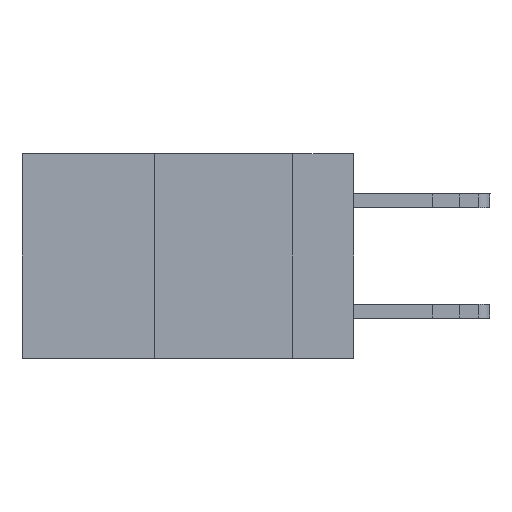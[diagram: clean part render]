
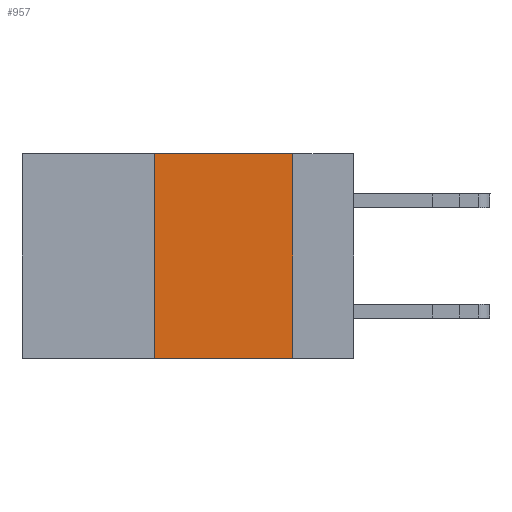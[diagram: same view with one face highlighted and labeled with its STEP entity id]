
A CAD part, left-side view. The second image highlights one B-rep face of the part: STEP entity #957.
In plain terms, the highlighted planar face has unit normal (-1, 0, 0).
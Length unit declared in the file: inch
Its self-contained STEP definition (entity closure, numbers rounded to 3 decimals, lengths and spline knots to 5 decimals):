
#957 = ADVANCED_FACE ( 'NONE', ( #14473 ), #7053, .F. ) ;
#1133 = CARTESIAN_POINT ( 'NONE',  ( 0., 0.36, 0. ) ) ;
#2918 = VERTEX_POINT ( 'NONE', #21353 ) ;
#3142 = EDGE_CURVE ( 'NONE', #7603, #15066, #15410, .T. ) ;
#4010 = EDGE_LOOP ( 'NONE', ( #4540, #5049, #11588, #8796 ) ) ;
#4540 = ORIENTED_EDGE ( 'NONE', *, *, #12472, .F. ) ;
#4547 = LINE ( 'NONE', #1133, #7385 ) ;
#4725 = DIRECTION ( 'NONE',  ( 0., 0., -1. ) ) ;
#4983 = CARTESIAN_POINT ( 'NONE',  ( 0., 0.36, 0. ) ) ;
#5049 = ORIENTED_EDGE ( 'NONE', *, *, #16550, .F. ) ;
#5548 = DIRECTION ( 'NONE',  ( 0., 0., 1. ) ) ;
#5970 = CARTESIAN_POINT ( 'NONE',  ( 0., 0.11, -0.37 ) ) ;
#6630 = VECTOR ( 'NONE', #7827, 39.37008 ) ;
#7053 = PLANE ( 'NONE',  #13541 ) ;
#7385 = VECTOR ( 'NONE', #5548, 39.37008 ) ;
#7603 = VERTEX_POINT ( 'NONE', #17558 ) ;
#7827 = DIRECTION ( 'NONE',  ( 0., -1., 0. ) ) ;
#8043 = VECTOR ( 'NONE', #4725, 39.37008 ) ;
#8620 = CARTESIAN_POINT ( 'NONE',  ( 0., 0.6, 0. ) ) ;
#8796 = ORIENTED_EDGE ( 'NONE', *, *, #3142, .T. ) ;
#9629 = CARTESIAN_POINT ( 'NONE',  ( 0., 0.6, 0. ) ) ;
#11544 = DIRECTION ( 'NONE',  ( 0., -1., 0. ) ) ;
#11588 = ORIENTED_EDGE ( 'NONE', *, *, #17045, .F. ) ;
#12472 = EDGE_CURVE ( 'NONE', #2918, #15066, #12533, .T. ) ;
#12533 = LINE ( 'NONE', #14823, #8043 ) ;
#13541 = AXIS2_PLACEMENT_3D ( 'NONE', #8620, #13663, #15583 ) ;
#13663 = DIRECTION ( 'NONE',  ( 1., 0., 0. ) ) ;
#14473 = FACE_OUTER_BOUND ( 'NONE', #4010, .T. ) ;
#14823 = CARTESIAN_POINT ( 'NONE',  ( 0., 0.11, 0. ) ) ;
#14886 = VECTOR ( 'NONE', #11544, 39.37008 ) ;
#15066 = VERTEX_POINT ( 'NONE', #5970 ) ;
#15377 = LINE ( 'NONE', #9629, #6630 ) ;
#15410 = LINE ( 'NONE', #19911, #14886 ) ;
#15583 = DIRECTION ( 'NONE',  ( 0., 0., -1. ) ) ;
#16550 = EDGE_CURVE ( 'NONE', #17274, #2918, #15377, .T. ) ;
#17045 = EDGE_CURVE ( 'NONE', #7603, #17274, #4547, .T. ) ;
#17274 = VERTEX_POINT ( 'NONE', #4983 ) ;
#17558 = CARTESIAN_POINT ( 'NONE',  ( 0., 0.36, -0.37 ) ) ;
#19911 = CARTESIAN_POINT ( 'NONE',  ( 0., 0.6, -0.37 ) ) ;
#21353 = CARTESIAN_POINT ( 'NONE',  ( 0., 0.11, 0. ) ) ;
